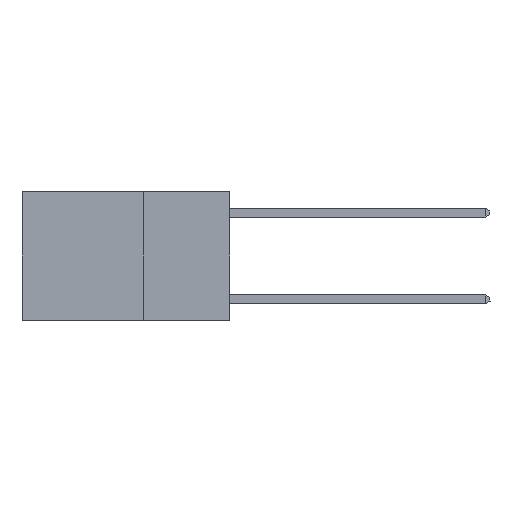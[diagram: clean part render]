
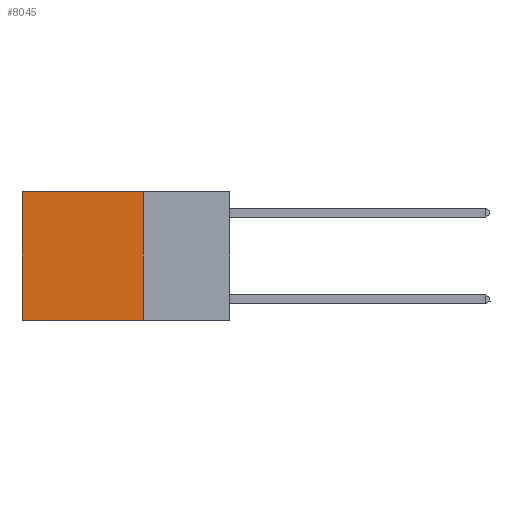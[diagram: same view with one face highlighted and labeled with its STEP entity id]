
A CAD part, left-side view. The second image highlights one B-rep face of the part: STEP entity #8045.
In plain terms, the highlighted planar face has unit normal (-1, 0, 0).
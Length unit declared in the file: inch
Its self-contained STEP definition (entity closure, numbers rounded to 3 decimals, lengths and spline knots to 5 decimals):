
#244 = DIRECTION ( 'NONE',  ( 0., 0., -1. ) ) ;
#1965 = VERTEX_POINT ( 'NONE', #7153 ) ;
#2273 = CARTESIAN_POINT ( 'NONE',  ( 0.2625, 0.6, 0. ) ) ;
#2373 = CARTESIAN_POINT ( 'NONE',  ( 0.2625, 0.6, -0.37 ) ) ;
#2872 = VECTOR ( 'NONE', #19200, 39.37008 ) ;
#3711 = EDGE_CURVE ( 'NONE', #1965, #17721, #6641, .T. ) ;
#3972 = CARTESIAN_POINT ( 'NONE',  ( 0.2625, 0.25, 0. ) ) ;
#4426 = ORIENTED_EDGE ( 'NONE', *, *, #12219, .T. ) ;
#4460 = LINE ( 'NONE', #2273, #9329 ) ;
#5983 = CARTESIAN_POINT ( 'NONE',  ( 0.2625, 0.25, 0. ) ) ;
#6641 = LINE ( 'NONE', #3972, #7944 ) ;
#7153 = CARTESIAN_POINT ( 'NONE',  ( 0.2625, 0.25, 0. ) ) ;
#7944 = VECTOR ( 'NONE', #16454, 39.37008 ) ;
#8041 = DIRECTION ( 'NONE',  ( 1., 0., 0. ) ) ;
#8045 = ADVANCED_FACE ( 'NONE', ( #8046 ), #18430, .F. ) ;
#8046 = FACE_OUTER_BOUND ( 'NONE', #20334, .T. ) ;
#9329 = VECTOR ( 'NONE', #244, 39.37008 ) ;
#10326 = ORIENTED_EDGE ( 'NONE', *, *, #3711, .T. ) ;
#10832 = CARTESIAN_POINT ( 'NONE',  ( 0.2625, 0.25, -0.37 ) ) ;
#11922 = CARTESIAN_POINT ( 'NONE',  ( 0.2625, 0.25, 0. ) ) ;
#12219 = EDGE_CURVE ( 'NONE', #17721, #14248, #4460, .T. ) ;
#12775 = ORIENTED_EDGE ( 'NONE', *, *, #13342, .F. ) ;
#13342 = EDGE_CURVE ( 'NONE', #1965, #23304, #15798, .T. ) ;
#14248 = VERTEX_POINT ( 'NONE', #2373 ) ;
#15798 = LINE ( 'NONE', #11922, #16459 ) ;
#16454 = DIRECTION ( 'NONE',  ( 0., 1., 0. ) ) ;
#16459 = VECTOR ( 'NONE', #26387, 39.37008 ) ;
#17721 = VERTEX_POINT ( 'NONE', #19481 ) ;
#18430 = PLANE ( 'NONE',  #26609 ) ;
#19200 = DIRECTION ( 'NONE',  ( 0., 1., 0. ) ) ;
#19366 = CARTESIAN_POINT ( 'NONE',  ( 0.2625, 0.25, -0.37 ) ) ;
#19481 = CARTESIAN_POINT ( 'NONE',  ( 0.2625, 0.6, 0. ) ) ;
#20334 = EDGE_LOOP ( 'NONE', ( #4426, #25821, #12775, #10326 ) ) ;
#22483 = EDGE_CURVE ( 'NONE', #23304, #14248, #25623, .T. ) ;
#22580 = DIRECTION ( 'NONE',  ( 0., 0., -1. ) ) ;
#23304 = VERTEX_POINT ( 'NONE', #19366 ) ;
#25623 = LINE ( 'NONE', #10832, #2872 ) ;
#25821 = ORIENTED_EDGE ( 'NONE', *, *, #22483, .F. ) ;
#26387 = DIRECTION ( 'NONE',  ( 0., 0., -1. ) ) ;
#26609 = AXIS2_PLACEMENT_3D ( 'NONE', #5983, #8041, #22580 ) ;
